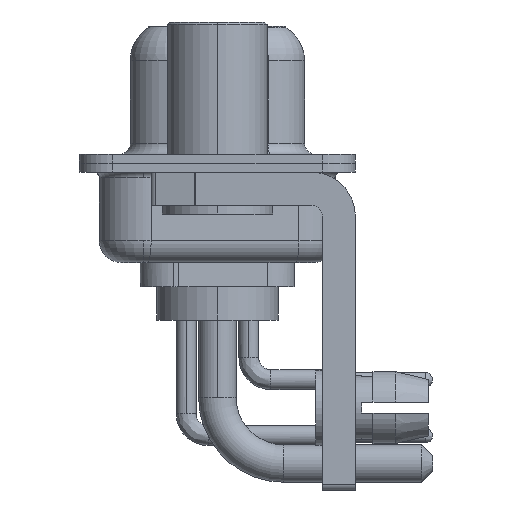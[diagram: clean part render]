
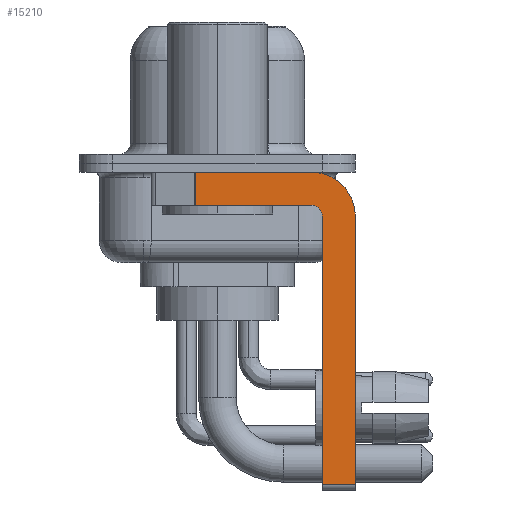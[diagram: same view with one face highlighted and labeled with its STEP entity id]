
A CAD part, left-side view. The second image highlights one B-rep face of the part: STEP entity #15210.
In plain terms, the highlighted planar face has unit normal (-1, 0, 0).
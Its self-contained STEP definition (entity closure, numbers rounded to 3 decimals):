
#725 = LINE ( 'NONE', #14827, #14544 ) ;
#760 = DIRECTION ( 'NONE',  ( 0., 0., -1. ) ) ;
#1207 = CARTESIAN_POINT ( 'NONE',  ( -2.9, -6.25, -2.4 ) ) ;
#1552 = LINE ( 'NONE', #1207, #21482 ) ;
#1839 = VECTOR ( 'NONE', #8126, 1000. ) ;
#1963 = DIRECTION ( 'NONE',  ( 0., 0., -1. ) ) ;
#2151 = AXIS2_PLACEMENT_3D ( 'NONE', #17917, #3714, #1963 ) ;
#2164 = EDGE_CURVE ( 'NONE', #6048, #14696, #22671, .T. ) ;
#2223 = DIRECTION ( 'NONE',  ( -1., 0., 0. ) ) ;
#2249 = DIRECTION ( 'NONE',  ( 0., 0., 1. ) ) ;
#2269 = CARTESIAN_POINT ( 'NONE',  ( -2.9, 3., -0.4 ) ) ;
#2572 = VERTEX_POINT ( 'NONE', #22294 ) ;
#3030 = LINE ( 'NONE', #20987, #19263 ) ;
#3714 = DIRECTION ( 'NONE',  ( 1., 0., 0. ) ) ;
#3829 = VECTOR ( 'NONE', #16604, 1000. ) ;
#4367 = LINE ( 'NONE', #2269, #3829 ) ;
#5334 = ORIENTED_EDGE ( 'NONE', *, *, #2164, .T. ) ;
#5685 = VERTEX_POINT ( 'NONE', #8523 ) ;
#6048 = VERTEX_POINT ( 'NONE', #18682 ) ;
#6080 = CARTESIAN_POINT ( 'NONE',  ( -2.9, -6.25, -14.55 ) ) ;
#6094 = EDGE_CURVE ( 'NONE', #15946, #2572, #4367, .T. ) ;
#6961 = VERTEX_POINT ( 'NONE', #10930 ) ;
#7397 = VERTEX_POINT ( 'NONE', #13010 ) ;
#7446 = ORIENTED_EDGE ( 'NONE', *, *, #16211, .F. ) ;
#8126 = DIRECTION ( 'NONE',  ( 0., -1., 0. ) ) ;
#8523 = CARTESIAN_POINT ( 'NONE',  ( -2.9, -4.75, -2.4 ) ) ;
#8635 = CARTESIAN_POINT ( 'NONE',  ( -2.9, -4.25, -2.4 ) ) ;
#8702 = ORIENTED_EDGE ( 'NONE', *, *, #13919, .F. ) ;
#9059 = CARTESIAN_POINT ( 'NONE',  ( -2.9, -4.25, -2.4 ) ) ;
#10098 = EDGE_CURVE ( 'NONE', #22432, #14696, #1552, .T. ) ;
#10278 = DIRECTION ( 'NONE',  ( 0., 0., -1. ) ) ;
#10477 = AXIS2_PLACEMENT_3D ( 'NONE', #8635, #19292, #10278 ) ;
#10593 = ORIENTED_EDGE ( 'NONE', *, *, #13368, .F. ) ;
#10930 = CARTESIAN_POINT ( 'NONE',  ( -2.9, 0.978, -1.9 ) ) ;
#11064 = DIRECTION ( 'NONE',  ( 0., 0., 1. ) ) ;
#11931 = CIRCLE ( 'NONE', #2151, 2. ) ;
#13010 = CARTESIAN_POINT ( 'NONE',  ( -2.9, -4.25, -1.9 ) ) ;
#13168 = VECTOR ( 'NONE', #22539, 1000. ) ;
#13368 = EDGE_CURVE ( 'NONE', #2572, #22432, #11931, .T. ) ;
#13919 = EDGE_CURVE ( 'NONE', #6048, #5685, #725, .T. ) ;
#13920 = FACE_OUTER_BOUND ( 'NONE', #17641, .T. ) ;
#14004 = DIRECTION ( 'NONE',  ( 0., 0., -1. ) ) ;
#14544 = VECTOR ( 'NONE', #2249, 1000. ) ;
#14696 = VERTEX_POINT ( 'NONE', #6080 ) ;
#14827 = CARTESIAN_POINT ( 'NONE',  ( -2.9, -4.75, -14.8 ) ) ;
#15210 = ADVANCED_FACE ( 'NONE', ( #13920 ), #18945, .F. ) ;
#15946 = VERTEX_POINT ( 'NONE', #16798 ) ;
#16211 = EDGE_CURVE ( 'NONE', #7397, #6961, #21320, .T. ) ;
#16604 = DIRECTION ( 'NONE',  ( 0., -1., 0. ) ) ;
#16798 = CARTESIAN_POINT ( 'NONE',  ( -2.9, 0.978, -0.4 ) ) ;
#17641 = EDGE_LOOP ( 'NONE', ( #21574, #20603, #7446, #17823, #8702, #5334, #22645, #10593 ) ) ;
#17823 = ORIENTED_EDGE ( 'NONE', *, *, #22031, .F. ) ;
#17917 = CARTESIAN_POINT ( 'NONE',  ( -2.9, -4.25, -2.4 ) ) ;
#18682 = CARTESIAN_POINT ( 'NONE',  ( -2.9, -4.75, -14.55 ) ) ;
#18945 = PLANE ( 'NONE',  #10477 ) ;
#19263 = VECTOR ( 'NONE', #760, 1000. ) ;
#19292 = DIRECTION ( 'NONE',  ( 1., 0., 0. ) ) ;
#19550 = CARTESIAN_POINT ( 'NONE',  ( -2.9, -4.25, -1.9 ) ) ;
#19611 = AXIS2_PLACEMENT_3D ( 'NONE', #9059, #2223, #11064 ) ;
#20603 = ORIENTED_EDGE ( 'NONE', *, *, #20974, .T. ) ;
#20677 = CARTESIAN_POINT ( 'NONE',  ( -2.9, -4.25, -14.55 ) ) ;
#20974 = EDGE_CURVE ( 'NONE', #15946, #6961, #3030, .T. ) ;
#20987 = CARTESIAN_POINT ( 'NONE',  ( -2.9, 0.978, -1.9 ) ) ;
#21320 = LINE ( 'NONE', #19550, #13168 ) ;
#21482 = VECTOR ( 'NONE', #14004, 1000. ) ;
#21570 = CARTESIAN_POINT ( 'NONE',  ( -2.9, -6.25, -2.4 ) ) ;
#21574 = ORIENTED_EDGE ( 'NONE', *, *, #6094, .F. ) ;
#22031 = EDGE_CURVE ( 'NONE', #5685, #7397, #22625, .T. ) ;
#22294 = CARTESIAN_POINT ( 'NONE',  ( -2.9, -4.25, -0.4 ) ) ;
#22432 = VERTEX_POINT ( 'NONE', #21570 ) ;
#22539 = DIRECTION ( 'NONE',  ( 0., 1., 0. ) ) ;
#22625 = CIRCLE ( 'NONE', #19611, 0.5 ) ;
#22645 = ORIENTED_EDGE ( 'NONE', *, *, #10098, .F. ) ;
#22671 = LINE ( 'NONE', #20677, #1839 ) ;
